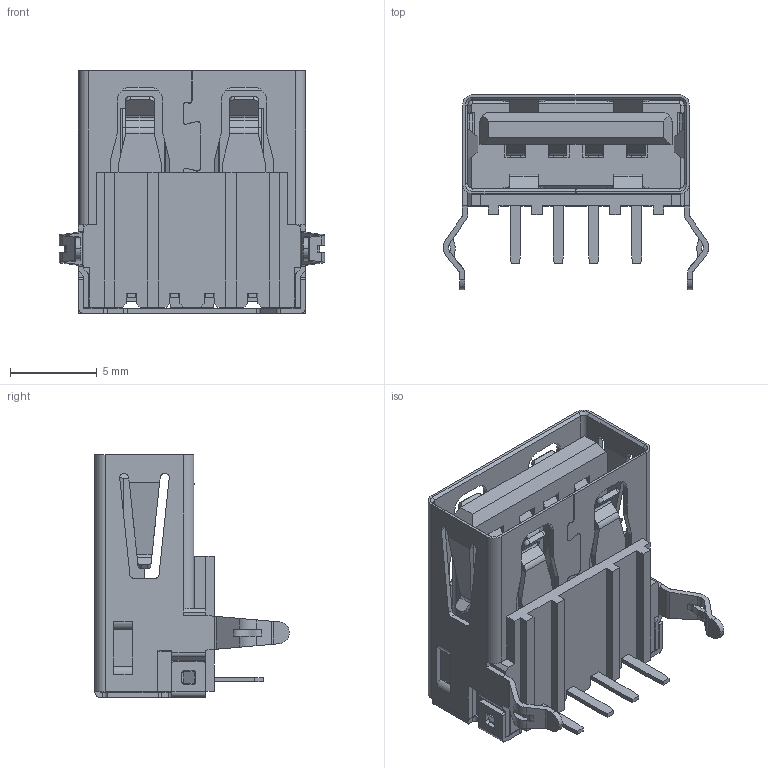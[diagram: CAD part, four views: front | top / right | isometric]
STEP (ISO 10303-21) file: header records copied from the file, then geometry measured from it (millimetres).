
FILE_DESCRIPTION (( 'STEP AP214' ), '1' );
FILE_NAME ('690A104-123-221.STEP', '2021-01-13T20:55:10', ( '' ), ( '' ), 'SwSTEP 2.0', 'SolidWorks 2020', '' );
FILE_SCHEMA (( 'AUTOMOTIVE_DESIGN' ));
Length unit declared in the file: millimetre
Products named in the file (4): 690A104-123-221; Shell 690A104-X23-22X; Insulator 690A104-X23-22X_Black; Contact 690A104-X23-22X
Assembly tree (6 placements, depth 2):
  690A104-123-221
    Shell 690A104-X23-22X
    Insulator 690A104-X23-22X_Black
    Contact 690A104-X23-22X  x4
Bounding box: 15.3 x 11.25 x 14 mm (x, y, z)
Volume: 573.9 mm3; surface area: 2129.5 mm2
Topology: 6 solids, 6 shells, 878 faces, 2593 edges, 1704 vertices
Faces by surface type: plane 658, cylinder 210, cone 6, bspline 4
Entity records: 23829 total; most frequent: CARTESIAN_POINT 4499, ORIENTED_EDGE 4220, DIRECTION 3775, EDGE_CURVE 2110, VECTOR 1707, LINE 1707, VERTEX_POINT 1386, AXIS2_PLACEMENT_3D 1034
